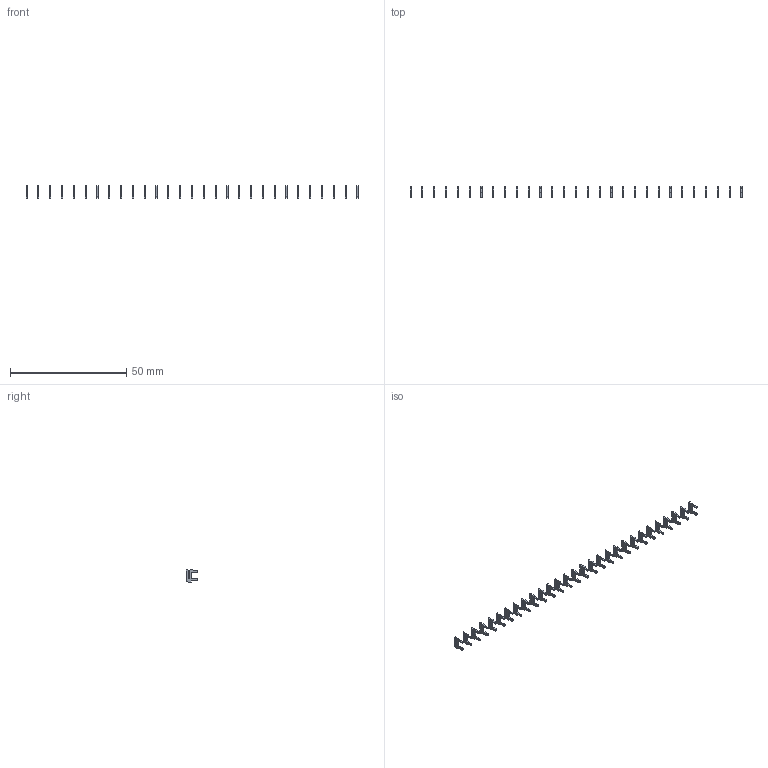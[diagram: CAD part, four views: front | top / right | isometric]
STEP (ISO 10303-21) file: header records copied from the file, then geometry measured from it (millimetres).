
FILE_DESCRIPTION (( 'STEP AP203' ), '1' );
FILE_NAME ('105-029-208-200.STEP', '2020-04-07T23:24:59', ( '' ), ( '' ), 'SwSTEP 2.0', 'SolidWorks 2016', '' );
FILE_SCHEMA (( 'CONFIG_CONTROL_DESIGN' ));
Length unit declared in the file: inch
Products named in the file (2): 100-290-001_100-290-208; 105-029-208-200
Assembly tree (29 placements, depth 2):
  105-029-208-200
    100-290-001_100-290-208  x29
Bounding box: 142.75 x 4.83 x 5.17 mm (x, y, z)
Volume: 199.5 mm3; surface area: 1232.4 mm2
Topology: 29 solids, 29 shells, 725 faces, 2001 edges, 1334 vertices
Faces by surface type: plane 638, cylinder 87
Entity records: 1885 total; most frequent: DIRECTION 189, CARTESIAN_POINT 172, ORIENTED_EDGE 138, EDGE_CURVE 69, DATE_AND_TIME 68, LOCAL_TIME 68, CALENDAR_DATE 68, COORDINATED_UNIVERSAL_TIME_OFFSET 68
